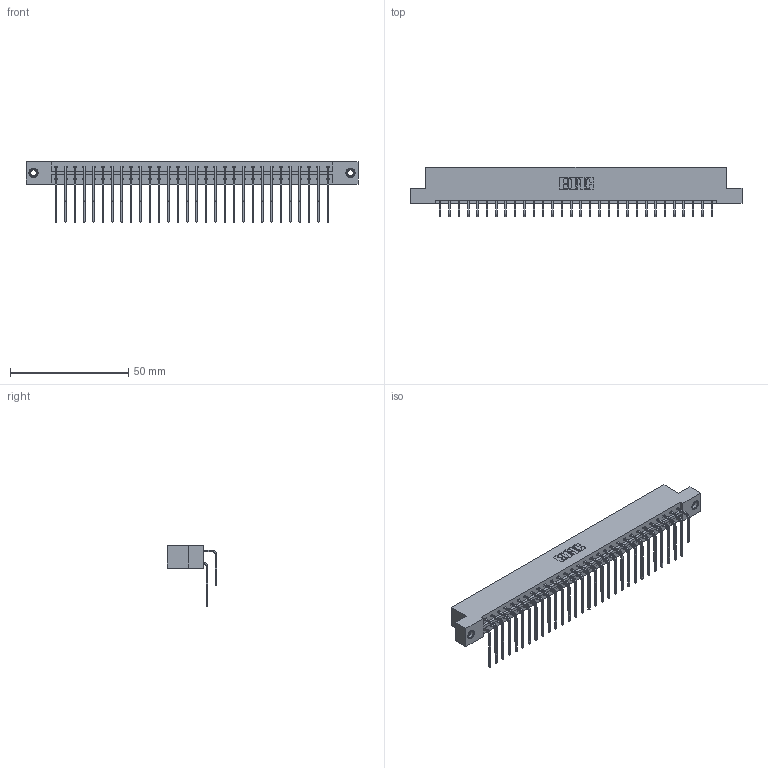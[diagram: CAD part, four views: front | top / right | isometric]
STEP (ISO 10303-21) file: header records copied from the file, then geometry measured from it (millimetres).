
FILE_DESCRIPTION (( 'STEP AP203' ), '1' );
FILE_NAME ('833-060-559-207.STEP', '2020-06-05T04:46:06', ( '' ), ( '' ), 'SwSTEP 2.0', 'SolidWorks 2020', '' );
FILE_SCHEMA (( 'CONFIG_CONTROL_DESIGN' ));
Length unit declared in the file: inch
Products named in the file (5): 345-292-001_559 Tail - 2; 833-060-559-207; 345-250-001_345-250-005-103; 833 Part_Flush - .156 Dia - TI; 345-292-001_558 559 Tail - 1
Assembly tree (63 placements, depth 2):
  833-060-559-207
    833 Part_Flush - .156 Dia - TI
    345-292-001_558 559 Tail - 1  x30
    345-292-001_559 Tail - 2  x30
    345-250-001_345-250-005-103  x2
Bounding box: 140.41 x 20.9 x 25.53 mm (x, y, z)
Volume: 14555.6 mm3; surface area: 18837.5 mm2
Topology: 63 solids, 63 shells, 3414 faces, 10107 edges, 6650 vertices
Faces by surface type: plane 2382, cylinder 1016, cone 12, torus 4
Entity records: 23822 total; most frequent: CARTESIAN_POINT 3996, ORIENTED_EDGE 3874, DIRECTION 3447, EDGE_CURVE 1937, LINE 1749, VECTOR 1749, VERTEX_POINT 1284, AXIS2_PLACEMENT_3D 849
